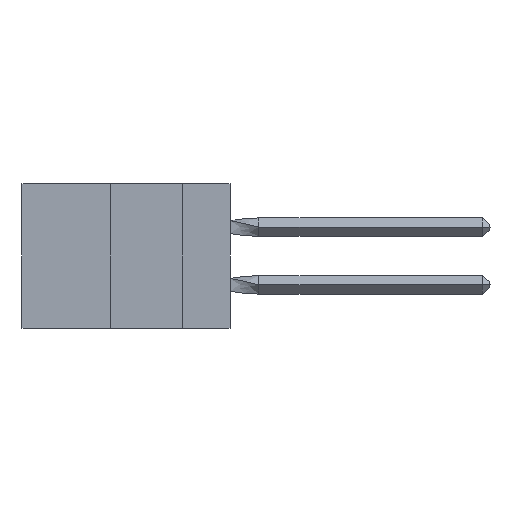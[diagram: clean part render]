
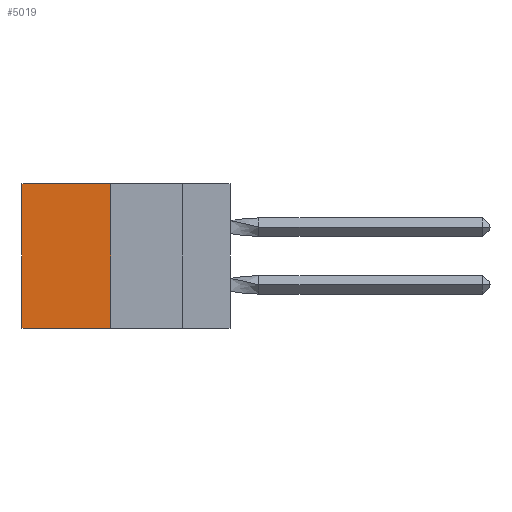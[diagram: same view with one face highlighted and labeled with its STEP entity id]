
A CAD part, left-side view. The second image highlights one B-rep face of the part: STEP entity #5019.
In plain terms, the highlighted planar face has unit normal (-1, 0, 0).
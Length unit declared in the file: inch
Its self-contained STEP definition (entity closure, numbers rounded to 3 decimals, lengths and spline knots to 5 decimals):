
#168 = VECTOR ( 'NONE', #4085, 39.37008 ) ;
#332 = LINE ( 'NONE', #11229, #168 ) ;
#1003 = DIRECTION ( 'NONE',  ( 0., 0., -1. ) ) ;
#1573 = EDGE_CURVE ( 'NONE', #2722, #3056, #14284, .T. ) ;
#1923 = DIRECTION ( 'NONE',  ( 0., 0., -1. ) ) ;
#2538 = EDGE_CURVE ( 'NONE', #11124, #3056, #7212, .T. ) ;
#2722 = VERTEX_POINT ( 'NONE', #12558 ) ;
#3056 = VERTEX_POINT ( 'NONE', #14505 ) ;
#3278 = PLANE ( 'NONE',  #10389 ) ;
#4085 = DIRECTION ( 'NONE',  ( 0., 1., 0. ) ) ;
#4209 = ORIENTED_EDGE ( 'NONE', *, *, #11975, .T. ) ;
#4905 = ORIENTED_EDGE ( 'NONE', *, *, #1573, .F. ) ;
#5019 = ADVANCED_FACE ( 'NONE', ( #10001 ), #3278, .F. ) ;
#5903 = CARTESIAN_POINT ( 'NONE',  ( 0.305, 0.72, 0. ) ) ;
#7212 = LINE ( 'NONE', #14640, #7927 ) ;
#7927 = VECTOR ( 'NONE', #1923, 39.37008 ) ;
#8030 = EDGE_LOOP ( 'NONE', ( #10683, #4905, #13844, #4209 ) ) ;
#8316 = DIRECTION ( 'NONE',  ( 0., 1., 0. ) ) ;
#9836 = VECTOR ( 'NONE', #14903, 39.37008 ) ;
#9849 = VERTEX_POINT ( 'NONE', #11539 ) ;
#10001 = FACE_OUTER_BOUND ( 'NONE', #8030, .T. ) ;
#10108 = CARTESIAN_POINT ( 'NONE',  ( 0.305, 0.413, -0.5 ) ) ;
#10389 = AXIS2_PLACEMENT_3D ( 'NONE', #10108, #11400, #1003 ) ;
#10683 = ORIENTED_EDGE ( 'NONE', *, *, #2538, .T. ) ;
#11124 = VERTEX_POINT ( 'NONE', #5903 ) ;
#11229 = CARTESIAN_POINT ( 'NONE',  ( 0.305, 0.413, 0. ) ) ;
#11313 = LINE ( 'NONE', #13750, #9836 ) ;
#11400 = DIRECTION ( 'NONE',  ( 1., 0., 0. ) ) ;
#11539 = CARTESIAN_POINT ( 'NONE',  ( 0.305, 0.413, 0. ) ) ;
#11975 = EDGE_CURVE ( 'NONE', #9849, #11124, #332, .T. ) ;
#12558 = CARTESIAN_POINT ( 'NONE',  ( 0.305, 0.413, -0.5 ) ) ;
#13750 = CARTESIAN_POINT ( 'NONE',  ( 0.305, 0.413, -0.5 ) ) ;
#13844 = ORIENTED_EDGE ( 'NONE', *, *, #14622, .F. ) ;
#13930 = VECTOR ( 'NONE', #8316, 39.37008 ) ;
#14155 = CARTESIAN_POINT ( 'NONE',  ( 0.305, 0.413, -0.5 ) ) ;
#14284 = LINE ( 'NONE', #14155, #13930 ) ;
#14505 = CARTESIAN_POINT ( 'NONE',  ( 0.305, 0.72, -0.5 ) ) ;
#14622 = EDGE_CURVE ( 'NONE', #9849, #2722, #11313, .T. ) ;
#14640 = CARTESIAN_POINT ( 'NONE',  ( 0.305, 0.72, -0.5 ) ) ;
#14903 = DIRECTION ( 'NONE',  ( 0., 0., -1. ) ) ;
